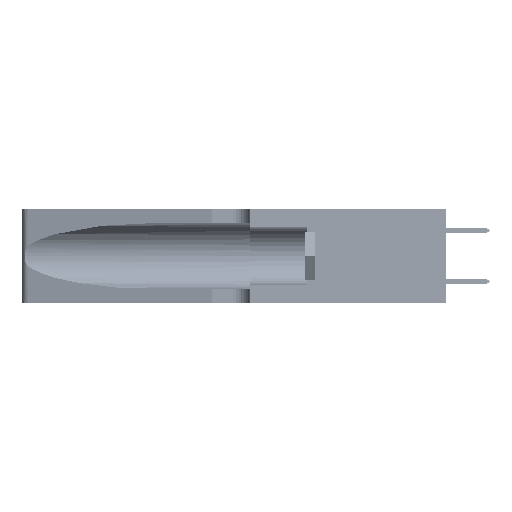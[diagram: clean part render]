
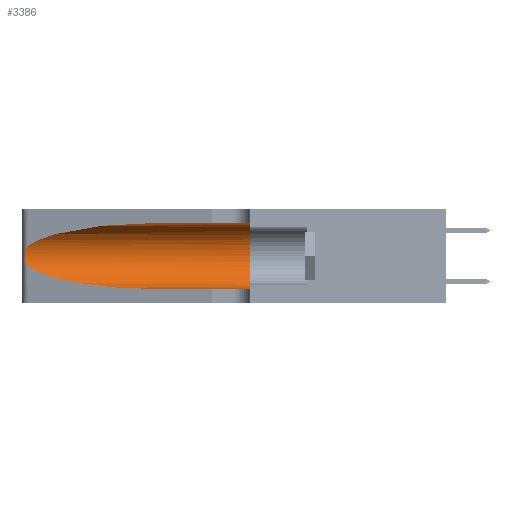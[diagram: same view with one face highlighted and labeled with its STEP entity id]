
A CAD part, left-side view. The second image highlights one B-rep face of the part: STEP entity #3386.
In plain terms, the highlighted cylindrical face has radius 3.308 mm (diameter 6.617 mm), a partial arc.
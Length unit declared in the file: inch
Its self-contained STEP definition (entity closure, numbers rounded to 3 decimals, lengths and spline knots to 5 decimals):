
#939 = CARTESIAN_POINT ( 'NONE',  ( 0.1305, 1.61858, 0.185 ) ) ;
#1227 = B_SPLINE_CURVE_WITH_KNOTS ( 'NONE', 3,
 ( #39234, #12692, #20371, #46774, #24166, #1379, #28001, #5210, #31808, #9027, #35590, #12851, #39406, #16699 ),
 .UNSPECIFIED., .F., .F.,
 ( 4, 2, 2, 2, 2, 2, 4 ),
 ( 0., 0.00027, 0.00053, 0.00107, 0.0016, 0.00187, 0.00214 ),
 .UNSPECIFIED. ) ;
#1379 = CARTESIAN_POINT ( 'NONE',  ( 0.26018, 1.23835, 0.19895 ) ) ;
#3040 = CARTESIAN_POINT ( 'NONE',  ( 0.1305, 0.35, 0.05475 ) ) ;
#3386 = ADVANCED_FACE ( 'NONE', ( #9580 ), #37487, .F. ) ;
#3545 = DIRECTION ( 'NONE',  ( 0., 1., 0. ) ) ;
#3615 = CARTESIAN_POINT ( 'NONE',  ( 0.25487, 1.22718, 0.14631 ) ) ;
#4681 = EDGE_CURVE ( 'NONE', #31942, #22165, #4746, .T. ) ;
#4746 = LINE ( 'NONE', #8828, #32697 ) ;
#5210 = CARTESIAN_POINT ( 'NONE',  ( 0.26075, 1.23896, 0.178 ) ) ;
#6985 = VERTEX_POINT ( 'NONE', #41149 ) ;
#7618 = CARTESIAN_POINT ( 'NONE',  ( 0.1305, 0.72297, 0.05475 ) ) ;
#8828 = CARTESIAN_POINT ( 'NONE',  ( 0.1305, 1.61858, 0.05475 ) ) ;
#9027 = CARTESIAN_POINT ( 'NONE',  ( 0.25856, 1.23593, 0.16098 ) ) ;
#9477 = CARTESIAN_POINT ( 'NONE',  ( 0.2373, 1.15595, 0.28018 ) ) ;
#9580 = FACE_OUTER_BOUND ( 'NONE', #25893, .T. ) ;
#11564 = AXIS2_PLACEMENT_3D ( 'NONE', #939, #31368, #38972 ) ;
#12692 = CARTESIAN_POINT ( 'NONE',  ( 0.25555, 1.22994, 0.2215 ) ) ;
#12851 = CARTESIAN_POINT ( 'NONE',  ( 0.25639, 1.23186, 0.15144 ) ) ;
#13304 = CARTESIAN_POINT ( 'NONE',  ( 0.18966, 0.96281, 0.31525 ) ) ;
#16452 = EDGE_CURVE ( 'NONE', #23251, #29443, #18935, .T. ) ;
#16699 = CARTESIAN_POINT ( 'NONE',  ( 0.25487, 1.22718, 0.14631 ) ) ;
#17148 = CARTESIAN_POINT ( 'NONE',  ( 0.25487, 1.22718, 0.22369 ) ) ;
#17688 = EDGE_CURVE ( 'NONE', #29443, #19903, #1227, .T. ) ;
#18935 =( BOUNDED_CURVE ( )  B_SPLINE_CURVE ( 3, ( #39836, #13304, #9477, #17148 ),
 .UNSPECIFIED., .F., .T. ) 
 B_SPLINE_CURVE_WITH_KNOTS ( ( 4, 4 ),
 ( 1.5708, 2.84003 ),
 .UNSPECIFIED. ) 
 CURVE ( )  GEOMETRIC_REPRESENTATION_ITEM ( )  RATIONAL_B_SPLINE_CURVE ( ( 1., 0.87, 0.87, 1. ) ) 
 REPRESENTATION_ITEM ( '' )  );
#19460 = CIRCLE ( 'NONE', #44521, 0.13025 ) ;
#19903 = VERTEX_POINT ( 'NONE', #20300 ) ;
#20300 = CARTESIAN_POINT ( 'NONE',  ( 0.25487, 1.22718, 0.14631 ) ) ;
#20371 = CARTESIAN_POINT ( 'NONE',  ( 0.25639, 1.23184, 0.21858 ) ) ;
#20559 = EDGE_CURVE ( 'NONE', #6985, #22165, #19460, .T. ) ;
#21158 = CARTESIAN_POINT ( 'NONE',  ( 0.25487, 1.22718, 0.22369 ) ) ;
#22165 = VERTEX_POINT ( 'NONE', #3040 ) ;
#23251 = VERTEX_POINT ( 'NONE', #43399 ) ;
#23948 = ORIENTED_EDGE ( 'NONE', *, *, #4681, .T. ) ;
#24166 = CARTESIAN_POINT ( 'NONE',  ( 0.25854, 1.2359, 0.20912 ) ) ;
#25850 = VECTOR ( 'NONE', #47342, 39.37008 ) ;
#25893 = EDGE_LOOP ( 'NONE', ( #34956, #48959, #26179, #23948, #31213, #41368 ) ) ;
#26179 = ORIENTED_EDGE ( 'NONE', *, *, #43888, .T. ) ;
#26350 = CARTESIAN_POINT ( 'NONE',  ( 0.1305, 0.35, 0.185 ) ) ;
#28001 = CARTESIAN_POINT ( 'NONE',  ( 0.26075, 1.23896, 0.19203 ) ) ;
#29443 = VERTEX_POINT ( 'NONE', #21158 ) ;
#30164 = DIRECTION ( 'NONE',  ( 0., 0., 1. ) ) ;
#30388 = CARTESIAN_POINT ( 'NONE',  ( 0.18966, 0.96281, 0.05475 ) ) ;
#31213 = ORIENTED_EDGE ( 'NONE', *, *, #20559, .F. ) ;
#31368 = DIRECTION ( 'NONE',  ( 0., -1., 0. ) ) ;
#31808 = CARTESIAN_POINT ( 'NONE',  ( 0.26017, 1.23833, 0.17102 ) ) ;
#31942 = VERTEX_POINT ( 'NONE', #40339 ) ;
#32199 = CARTESIAN_POINT ( 'NONE',  ( 0.1305, 1.61858, 0.31525 ) ) ;
#32697 = VECTOR ( 'NONE', #35388, 39.37008 ) ;
#34956 = ORIENTED_EDGE ( 'NONE', *, *, #16452, .T. ) ;
#35388 = DIRECTION ( 'NONE',  ( 0., -1., 0. ) ) ;
#35590 = CARTESIAN_POINT ( 'NONE',  ( 0.25789, 1.23486, 0.15765 ) ) ;
#36830 = EDGE_CURVE ( 'NONE', #23251, #6985, #47088, .T. ) ;
#37487 = CYLINDRICAL_SURFACE ( 'NONE', #11564, 0.13025 ) ;
#37848 = CARTESIAN_POINT ( 'NONE',  ( 0.2373, 1.15595, 0.08982 ) ) ;
#38071 =( BOUNDED_CURVE ( )  B_SPLINE_CURVE ( 3, ( #3615, #37848, #30388, #7618 ),
 .UNSPECIFIED., .F., .T. ) 
 B_SPLINE_CURVE_WITH_KNOTS ( ( 4, 4 ),
 ( 3.44316, 4.71239 ),
 .UNSPECIFIED. ) 
 CURVE ( )  GEOMETRIC_REPRESENTATION_ITEM ( )  RATIONAL_B_SPLINE_CURVE ( ( 1., 0.87, 0.87, 1. ) ) 
 REPRESENTATION_ITEM ( '' )  );
#38972 = DIRECTION ( 'NONE',  ( 0., 0., -1. ) ) ;
#39234 = CARTESIAN_POINT ( 'NONE',  ( 0.25487, 1.22718, 0.22369 ) ) ;
#39406 = CARTESIAN_POINT ( 'NONE',  ( 0.25555, 1.22993, 0.14849 ) ) ;
#39836 = CARTESIAN_POINT ( 'NONE',  ( 0.1305, 0.72297, 0.31525 ) ) ;
#40339 = CARTESIAN_POINT ( 'NONE',  ( 0.1305, 0.72297, 0.05475 ) ) ;
#41149 = CARTESIAN_POINT ( 'NONE',  ( 0.1305, 0.35, 0.31525 ) ) ;
#41368 = ORIENTED_EDGE ( 'NONE', *, *, #36830, .F. ) ;
#43399 = CARTESIAN_POINT ( 'NONE',  ( 0.1305, 0.72297, 0.31525 ) ) ;
#43888 = EDGE_CURVE ( 'NONE', #19903, #31942, #38071, .T. ) ;
#44521 = AXIS2_PLACEMENT_3D ( 'NONE', #26350, #3545, #30164 ) ;
#46774 = CARTESIAN_POINT ( 'NONE',  ( 0.25787, 1.23484, 0.2124 ) ) ;
#47088 = LINE ( 'NONE', #32199, #25850 ) ;
#47342 = DIRECTION ( 'NONE',  ( 0., -1., 0. ) ) ;
#48959 = ORIENTED_EDGE ( 'NONE', *, *, #17688, .T. ) ;
